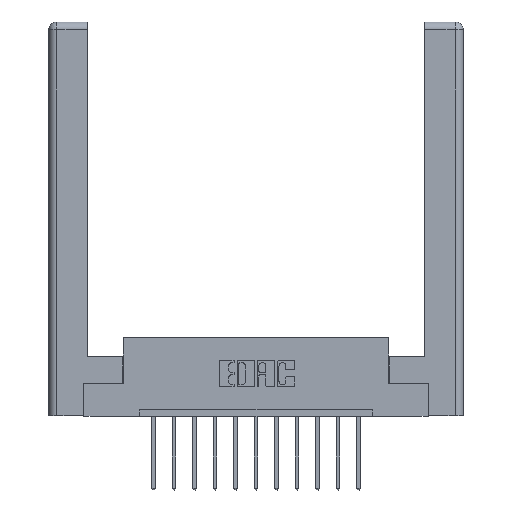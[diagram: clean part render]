
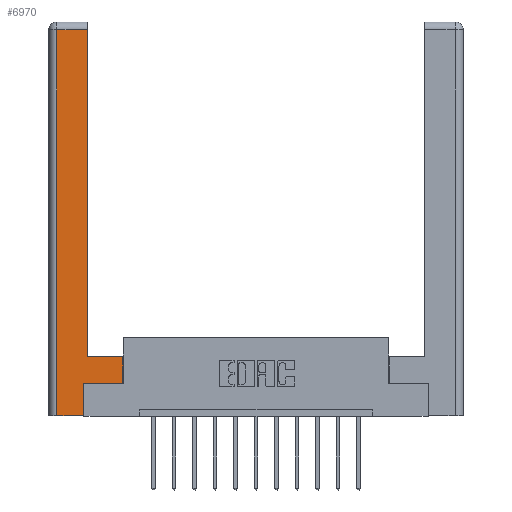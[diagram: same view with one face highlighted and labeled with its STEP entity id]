
A CAD part, top view. The second image highlights one B-rep face of the part: STEP entity #6970.
In plain terms, the highlighted planar face has unit normal (0, 0, 1).
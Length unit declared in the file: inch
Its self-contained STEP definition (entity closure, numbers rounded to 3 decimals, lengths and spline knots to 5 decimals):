
#27 = LINE ( 'NONE', #11711, #1618 ) ;
#134 = ORIENTED_EDGE ( 'NONE', *, *, #14090, .T. ) ;
#346 = CARTESIAN_POINT ( 'NONE',  ( 0.265, 0., 0. ) ) ;
#1027 = CARTESIAN_POINT ( 'NONE',  ( 0.265, 0.245, 0. ) ) ;
#1058 = CARTESIAN_POINT ( 'NONE',  ( 0.565, 0.245, 0. ) ) ;
#1130 = VECTOR ( 'NONE', #11136, 39.37008 ) ;
#1183 = LINE ( 'NONE', #14186, #13898 ) ;
#1617 = DIRECTION ( 'NONE',  ( 0., 1., 0. ) ) ;
#1618 = VECTOR ( 'NONE', #4832, 39.37008 ) ;
#1792 = EDGE_CURVE ( 'NONE', #10797, #10088, #8054, .T. ) ;
#2136 = VECTOR ( 'NONE', #5825, 39.37008 ) ;
#2223 = PLANE ( 'NONE',  #7674 ) ;
#2531 = CARTESIAN_POINT ( 'NONE',  ( 0.295, 3., 0. ) ) ;
#3065 = CARTESIAN_POINT ( 'NONE',  ( 0.0615, 0., 0. ) ) ;
#3392 = VERTEX_POINT ( 'NONE', #346 ) ;
#3549 = EDGE_CURVE ( 'NONE', #3629, #4708, #13580, .T. ) ;
#3585 = DIRECTION ( 'NONE',  ( 0., 0., -1. ) ) ;
#3629 = VERTEX_POINT ( 'NONE', #1027 ) ;
#3830 = ORIENTED_EDGE ( 'NONE', *, *, #5389, .T. ) ;
#4027 = LINE ( 'NONE', #7304, #12948 ) ;
#4256 = FACE_OUTER_BOUND ( 'NONE', #5476, .T. ) ;
#4323 = CARTESIAN_POINT ( 'NONE',  ( 0.265, 0., 0. ) ) ;
#4483 = DIRECTION ( 'NONE',  ( 1., 0., 0. ) ) ;
#4708 = VERTEX_POINT ( 'NONE', #1058 ) ;
#4831 = EDGE_CURVE ( 'NONE', #10088, #13609, #14624, .T. ) ;
#4832 = DIRECTION ( 'NONE',  ( 0., -1., 0. ) ) ;
#5338 = CARTESIAN_POINT ( 'NONE',  ( 0.295, 2.94, 0. ) ) ;
#5389 = EDGE_CURVE ( 'NONE', #3392, #3629, #4027, .T. ) ;
#5476 = EDGE_LOOP ( 'NONE', ( #8980, #9354, #9510, #7887, #3830, #14538, #134, #7179 ) ) ;
#5697 = CARTESIAN_POINT ( 'NONE',  ( 0.295, 0.45, 0. ) ) ;
#5746 = CARTESIAN_POINT ( 'NONE',  ( 0., 0., 0. ) ) ;
#5825 = DIRECTION ( 'NONE',  ( -1., 0., 0. ) ) ;
#5868 = VECTOR ( 'NONE', #4483, 39.37008 ) ;
#6416 = CARTESIAN_POINT ( 'NONE',  ( 0.0615, 2.94, 0. ) ) ;
#6970 = ADVANCED_FACE ( 'NONE', ( #4256 ), #2223, .F. ) ;
#7179 = ORIENTED_EDGE ( 'NONE', *, *, #1792, .T. ) ;
#7225 = VERTEX_POINT ( 'NONE', #6416 ) ;
#7304 = CARTESIAN_POINT ( 'NONE',  ( 0.265, 0.245, 0. ) ) ;
#7674 = AXIS2_PLACEMENT_3D ( 'NONE', #5746, #3585, #12614 ) ;
#7887 = ORIENTED_EDGE ( 'NONE', *, *, #9175, .T. ) ;
#8027 = CARTESIAN_POINT ( 'NONE',  ( 0.565, 0.45, 0. ) ) ;
#8054 = LINE ( 'NONE', #12692, #2136 ) ;
#8267 = DIRECTION ( 'NONE',  ( 0., 1., 0. ) ) ;
#8556 = DIRECTION ( 'NONE',  ( 0., 1., 0. ) ) ;
#8980 = ORIENTED_EDGE ( 'NONE', *, *, #4831, .T. ) ;
#9175 = EDGE_CURVE ( 'NONE', #13620, #3392, #13693, .T. ) ;
#9354 = ORIENTED_EDGE ( 'NONE', *, *, #12449, .T. ) ;
#9453 = VECTOR ( 'NONE', #13807, 39.37008 ) ;
#9510 = ORIENTED_EDGE ( 'NONE', *, *, #10906, .T. ) ;
#10041 = CARTESIAN_POINT ( 'NONE',  ( 0.565, 0.245, 0. ) ) ;
#10088 = VERTEX_POINT ( 'NONE', #5697 ) ;
#10126 = VECTOR ( 'NONE', #8267, 39.37008 ) ;
#10797 = VERTEX_POINT ( 'NONE', #8027 ) ;
#10906 = EDGE_CURVE ( 'NONE', #7225, #13620, #27, .T. ) ;
#11136 = DIRECTION ( 'NONE',  ( 1., 0., 0. ) ) ;
#11548 = CARTESIAN_POINT ( 'NONE',  ( 0.0615, 2.94, 0. ) ) ;
#11711 = CARTESIAN_POINT ( 'NONE',  ( 0.0615, 0., 0. ) ) ;
#12449 = EDGE_CURVE ( 'NONE', #13609, #7225, #12514, .T. ) ;
#12514 = LINE ( 'NONE', #11548, #9453 ) ;
#12614 = DIRECTION ( 'NONE',  ( -1., 0., 0. ) ) ;
#12692 = CARTESIAN_POINT ( 'NONE',  ( 0.295, 0.45, 0. ) ) ;
#12948 = VECTOR ( 'NONE', #1617, 39.37008 ) ;
#13580 = LINE ( 'NONE', #10041, #5868 ) ;
#13609 = VERTEX_POINT ( 'NONE', #5338 ) ;
#13620 = VERTEX_POINT ( 'NONE', #3065 ) ;
#13693 = LINE ( 'NONE', #4323, #1130 ) ;
#13807 = DIRECTION ( 'NONE',  ( -1., 0., 0. ) ) ;
#13898 = VECTOR ( 'NONE', #8556, 39.37008 ) ;
#14090 = EDGE_CURVE ( 'NONE', #4708, #10797, #1183, .T. ) ;
#14186 = CARTESIAN_POINT ( 'NONE',  ( 0.565, 0.45, 0. ) ) ;
#14538 = ORIENTED_EDGE ( 'NONE', *, *, #3549, .T. ) ;
#14624 = LINE ( 'NONE', #2531, #10126 ) ;
